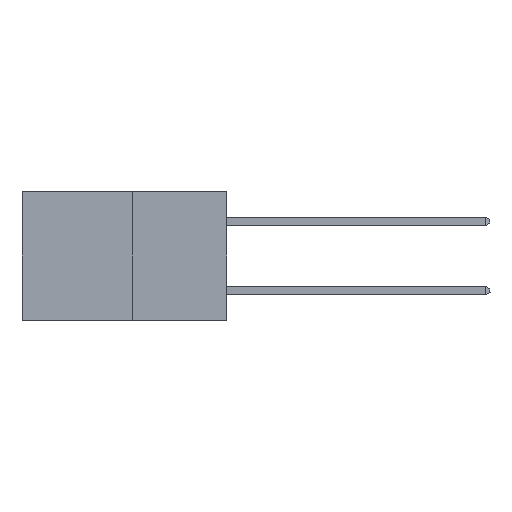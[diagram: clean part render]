
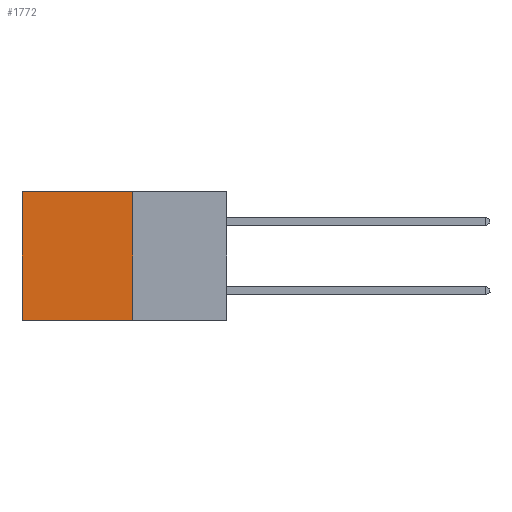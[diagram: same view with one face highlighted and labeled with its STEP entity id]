
A CAD part, left-side view. The second image highlights one B-rep face of the part: STEP entity #1772.
In plain terms, the highlighted planar face has unit normal (-1, 0, 0).
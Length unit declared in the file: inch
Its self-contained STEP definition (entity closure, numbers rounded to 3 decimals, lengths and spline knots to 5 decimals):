
#373 = LINE ( 'NONE', #5791, #592 ) ;
#451 = CARTESIAN_POINT ( 'NONE',  ( 0.277, 0.59, -0.37 ) ) ;
#592 = VECTOR ( 'NONE', #6700, 39.37008 ) ;
#661 = ORIENTED_EDGE ( 'NONE', *, *, #1504, .F. ) ;
#859 = DIRECTION ( 'NONE',  ( 0., 0., -1. ) ) ;
#864 = VERTEX_POINT ( 'NONE', #5632 ) ;
#1504 = EDGE_CURVE ( 'NONE', #864, #7798, #373, .T. ) ;
#1547 = VECTOR ( 'NONE', #859, 39.37008 ) ;
#1658 = CARTESIAN_POINT ( 'NONE',  ( 0.277, 0.59, -0.37 ) ) ;
#1772 = ADVANCED_FACE ( 'NONE', ( #8173 ), #7509, .F. ) ;
#1902 = EDGE_CURVE ( 'NONE', #7046, #864, #5619, .T. ) ;
#2018 = EDGE_CURVE ( 'NONE', #6459, #7798, #3929, .T. ) ;
#2109 = ORIENTED_EDGE ( 'NONE', *, *, #2018, .T. ) ;
#2119 = EDGE_CURVE ( 'NONE', #7046, #6459, #3026, .T. ) ;
#2731 = VECTOR ( 'NONE', #5609, 39.37008 ) ;
#3026 = LINE ( 'NONE', #6365, #2731 ) ;
#3661 = ORIENTED_EDGE ( 'NONE', *, *, #1902, .F. ) ;
#3929 = LINE ( 'NONE', #1658, #7291 ) ;
#4014 = CARTESIAN_POINT ( 'NONE',  ( 0.277, 0.59, 0. ) ) ;
#4280 = DIRECTION ( 'NONE',  ( 0., 0., -1. ) ) ;
#4764 = AXIS2_PLACEMENT_3D ( 'NONE', #7233, #8799, #4280 ) ;
#5609 = DIRECTION ( 'NONE',  ( 0., 1., 0. ) ) ;
#5619 = LINE ( 'NONE', #7763, #1547 ) ;
#5632 = CARTESIAN_POINT ( 'NONE',  ( 0.277, 0.27, -0.37 ) ) ;
#5791 = CARTESIAN_POINT ( 'NONE',  ( 0.277, 0.27, -0.37 ) ) ;
#6365 = CARTESIAN_POINT ( 'NONE',  ( 0.277, 0.27, 0. ) ) ;
#6459 = VERTEX_POINT ( 'NONE', #4014 ) ;
#6700 = DIRECTION ( 'NONE',  ( 0., 1., 0. ) ) ;
#7046 = VERTEX_POINT ( 'NONE', #7138 ) ;
#7138 = CARTESIAN_POINT ( 'NONE',  ( 0.277, 0.27, 0. ) ) ;
#7233 = CARTESIAN_POINT ( 'NONE',  ( 0.277, 0.27, -0.37 ) ) ;
#7291 = VECTOR ( 'NONE', #7754, 39.37008 ) ;
#7509 = PLANE ( 'NONE',  #4764 ) ;
#7754 = DIRECTION ( 'NONE',  ( 0., 0., -1. ) ) ;
#7763 = CARTESIAN_POINT ( 'NONE',  ( 0.277, 0.27, -0.37 ) ) ;
#7798 = VERTEX_POINT ( 'NONE', #451 ) ;
#7957 = EDGE_LOOP ( 'NONE', ( #2109, #661, #3661, #7973 ) ) ;
#7973 = ORIENTED_EDGE ( 'NONE', *, *, #2119, .T. ) ;
#8173 = FACE_OUTER_BOUND ( 'NONE', #7957, .T. ) ;
#8799 = DIRECTION ( 'NONE',  ( 1., 0., 0. ) ) ;
